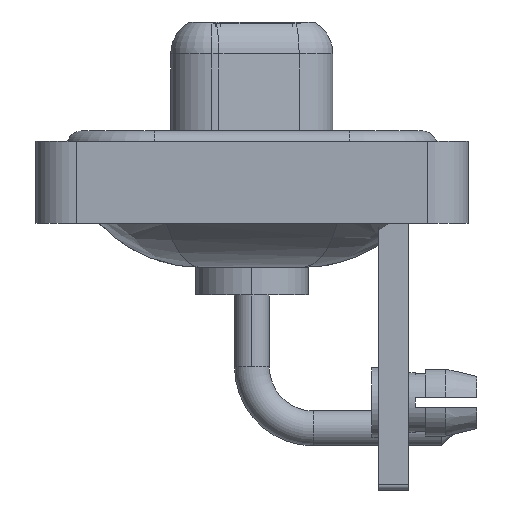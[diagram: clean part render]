
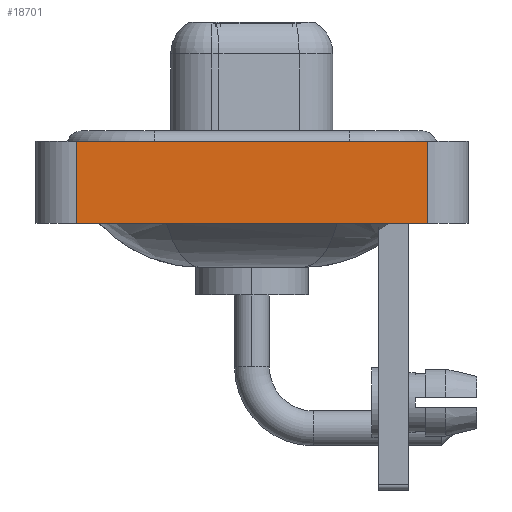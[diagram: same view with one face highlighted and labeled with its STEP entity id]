
A CAD part, left-side view. The second image highlights one B-rep face of the part: STEP entity #18701.
In plain terms, the highlighted planar face has unit normal (-1, 0, 0).
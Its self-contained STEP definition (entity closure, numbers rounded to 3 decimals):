
#462 = PLANE ( 'NONE',  #7931 ) ;
#1129 = EDGE_CURVE ( 'NONE', #14333, #11861, #10783, .T. ) ;
#1246 = VECTOR ( 'NONE', #13114, 1000. ) ;
#1371 = VERTEX_POINT ( 'NONE', #7823 ) ;
#1793 = CARTESIAN_POINT ( 'NONE',  ( -7.35, 8.55, -3.6 ) ) ;
#2824 = ORIENTED_EDGE ( 'NONE', *, *, #1129, .T. ) ;
#3056 = CARTESIAN_POINT ( 'NONE',  ( -7.35, -8.55, 0.4 ) ) ;
#4579 = EDGE_CURVE ( 'NONE', #1371, #14333, #4644, .T. ) ;
#4644 = LINE ( 'NONE', #7808, #14519 ) ;
#4943 = DIRECTION ( 'NONE',  ( 0., -1., 0. ) ) ;
#4981 = CARTESIAN_POINT ( 'NONE',  ( -7.35, -8.55, -3.6 ) ) ;
#5923 = LINE ( 'NONE', #1793, #1246 ) ;
#5960 = CARTESIAN_POINT ( 'NONE',  ( -7.35, -8.55, 0.4 ) ) ;
#6032 = DIRECTION ( 'NONE',  ( -1., 0., 0. ) ) ;
#7028 = CARTESIAN_POINT ( 'NONE',  ( -7.35, 8.55, 0.4 ) ) ;
#7662 = FACE_OUTER_BOUND ( 'NONE', #11678, .T. ) ;
#7808 = CARTESIAN_POINT ( 'NONE',  ( -7.35, -8.55, -3.6 ) ) ;
#7823 = CARTESIAN_POINT ( 'NONE',  ( -7.35, 8.55, -3.6 ) ) ;
#7931 = AXIS2_PLACEMENT_3D ( 'NONE', #4981, #6032, #12161 ) ;
#9963 = DIRECTION ( 'NONE',  ( 0., -1., 0. ) ) ;
#10081 = ORIENTED_EDGE ( 'NONE', *, *, #4579, .T. ) ;
#10783 = LINE ( 'NONE', #12317, #15526 ) ;
#11678 = EDGE_LOOP ( 'NONE', ( #2824, #14128, #17731, #10081 ) ) ;
#11861 = VERTEX_POINT ( 'NONE', #3056 ) ;
#12161 = DIRECTION ( 'NONE',  ( 0., 0., 1. ) ) ;
#12253 = EDGE_CURVE ( 'NONE', #1371, #15327, #5923, .T. ) ;
#12317 = CARTESIAN_POINT ( 'NONE',  ( -7.35, -8.55, -3.6 ) ) ;
#12610 = CARTESIAN_POINT ( 'NONE',  ( -7.35, -8.55, -3.6 ) ) ;
#13114 = DIRECTION ( 'NONE',  ( 0., 0., 1. ) ) ;
#13150 = LINE ( 'NONE', #5960, #13984 ) ;
#13984 = VECTOR ( 'NONE', #9963, 1000. ) ;
#14128 = ORIENTED_EDGE ( 'NONE', *, *, #15435, .F. ) ;
#14333 = VERTEX_POINT ( 'NONE', #12610 ) ;
#14519 = VECTOR ( 'NONE', #4943, 1000. ) ;
#15327 = VERTEX_POINT ( 'NONE', #7028 ) ;
#15435 = EDGE_CURVE ( 'NONE', #15327, #11861, #13150, .T. ) ;
#15473 = DIRECTION ( 'NONE',  ( 0., 0., 1. ) ) ;
#15526 = VECTOR ( 'NONE', #15473, 1000. ) ;
#17731 = ORIENTED_EDGE ( 'NONE', *, *, #12253, .F. ) ;
#18701 = ADVANCED_FACE ( 'NONE', ( #7662 ), #462, .T. ) ;
